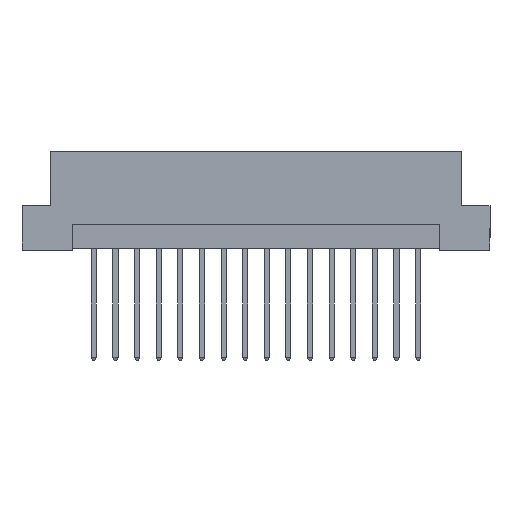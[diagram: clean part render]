
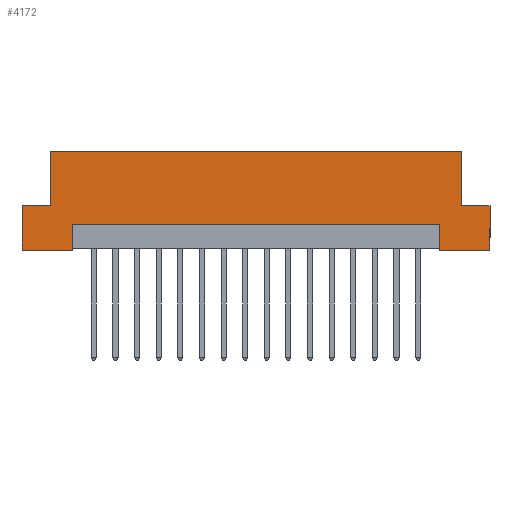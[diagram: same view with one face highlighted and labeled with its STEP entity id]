
A CAD part, front view. The second image highlights one B-rep face of the part: STEP entity #4172.
In plain terms, the highlighted planar face has unit normal (0, -1, 0).
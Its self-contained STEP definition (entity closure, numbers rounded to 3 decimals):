
#168 = CARTESIAN_POINT ( 'NONE',  ( -27.5, -4.3, 5.2 ) ) ;
#171 = VERTEX_POINT ( 'NONE', #2007 ) ;
#203 = CARTESIAN_POINT ( 'NONE',  ( 24.2, -4.3, 11.6 ) ) ;
#214 = EDGE_CURVE ( 'NONE', #5362, #229, #720, .T. ) ;
#229 = VERTEX_POINT ( 'NONE', #881 ) ;
#248 = VECTOR ( 'NONE', #6927, 1000. ) ;
#317 = CARTESIAN_POINT ( 'NONE',  ( -24.2, -4.3, 5.2 ) ) ;
#432 = EDGE_CURVE ( 'NONE', #5362, #6430, #910, .T. ) ;
#439 = ORIENTED_EDGE ( 'NONE', *, *, #6250, .T. ) ;
#578 = CARTESIAN_POINT ( 'NONE',  ( 21.6, -4.3, 0. ) ) ;
#686 = VECTOR ( 'NONE', #3645, 1000. ) ;
#720 = LINE ( 'NONE', #3054, #4377 ) ;
#773 = DIRECTION ( 'NONE',  ( 0., 0., 1. ) ) ;
#783 = LINE ( 'NONE', #5378, #5817 ) ;
#818 = PLANE ( 'NONE',  #4997 ) ;
#843 = EDGE_LOOP ( 'NONE', ( #439, #2009, #5413, #3270, #1506, #2650, #2389, #6124, #3688, #930, #3277, #5646 ) ) ;
#881 = CARTESIAN_POINT ( 'NONE',  ( 27.5, -4.3, 5.2 ) ) ;
#910 = LINE ( 'NONE', #3212, #1143 ) ;
#930 = ORIENTED_EDGE ( 'NONE', *, *, #5732, .T. ) ;
#951 = VERTEX_POINT ( 'NONE', #3939 ) ;
#1006 = CARTESIAN_POINT ( 'NONE',  ( -24.2, -4.3, 5.2 ) ) ;
#1043 = VERTEX_POINT ( 'NONE', #578 ) ;
#1130 = LINE ( 'NONE', #5734, #5064 ) ;
#1141 = LINE ( 'NONE', #3323, #6011 ) ;
#1143 = VECTOR ( 'NONE', #3805, 1000. ) ;
#1381 = VERTEX_POINT ( 'NONE', #5130 ) ;
#1394 = CARTESIAN_POINT ( 'NONE',  ( 27.5, -4.3, 0. ) ) ;
#1400 = FACE_OUTER_BOUND ( 'NONE', #843, .T. ) ;
#1461 = LINE ( 'NONE', #1394, #1472 ) ;
#1472 = VECTOR ( 'NONE', #3111, 1000. ) ;
#1506 = ORIENTED_EDGE ( 'NONE', *, *, #214, .F. ) ;
#1571 = VERTEX_POINT ( 'NONE', #1882 ) ;
#1882 = CARTESIAN_POINT ( 'NONE',  ( -24.2, -4.3, 11.6 ) ) ;
#2007 = CARTESIAN_POINT ( 'NONE',  ( -21.6, -4.3, 3. ) ) ;
#2009 = ORIENTED_EDGE ( 'NONE', *, *, #4235, .F. ) ;
#2164 = EDGE_CURVE ( 'NONE', #2628, #4800, #5532, .T. ) ;
#2256 = DIRECTION ( 'NONE',  ( 0., 0., -1. ) ) ;
#2317 = LINE ( 'NONE', #4165, #248 ) ;
#2388 = DIRECTION ( 'NONE',  ( 0., 0., -1. ) ) ;
#2389 = ORIENTED_EDGE ( 'NONE', *, *, #6824, .F. ) ;
#2508 = DIRECTION ( 'NONE',  ( 0., 0., 1. ) ) ;
#2518 = CARTESIAN_POINT ( 'NONE',  ( -21.6, -4.3, 0.2 ) ) ;
#2628 = VERTEX_POINT ( 'NONE', #168 ) ;
#2641 = LINE ( 'NONE', #2518, #4529 ) ;
#2650 = ORIENTED_EDGE ( 'NONE', *, *, #432, .T. ) ;
#2858 = EDGE_CURVE ( 'NONE', #3959, #1381, #6196, .T. ) ;
#2881 = CARTESIAN_POINT ( 'NONE',  ( 27.5, -4.3, 11.6 ) ) ;
#3054 = CARTESIAN_POINT ( 'NONE',  ( 27.5, -4.3, 5.2 ) ) ;
#3111 = DIRECTION ( 'NONE',  ( 1., 0., 0. ) ) ;
#3212 = CARTESIAN_POINT ( 'NONE',  ( 24.2, -4.3, 5.2 ) ) ;
#3270 = ORIENTED_EDGE ( 'NONE', *, *, #4976, .F. ) ;
#3272 = DIRECTION ( 'NONE',  ( 1., 0., 0. ) ) ;
#3277 = ORIENTED_EDGE ( 'NONE', *, *, #2858, .T. ) ;
#3323 = CARTESIAN_POINT ( 'NONE',  ( -27.5, -4.3, 11.6 ) ) ;
#3645 = DIRECTION ( 'NONE',  ( 1., 0., 0. ) ) ;
#3646 = EDGE_CURVE ( 'NONE', #171, #1381, #2641, .T. ) ;
#3688 = ORIENTED_EDGE ( 'NONE', *, *, #2164, .F. ) ;
#3757 = DIRECTION ( 'NONE',  ( 0., 1., 0. ) ) ;
#3801 = DIRECTION ( 'NONE',  ( 0., 0., -1. ) ) ;
#3805 = DIRECTION ( 'NONE',  ( 0., 0., 1. ) ) ;
#3939 = CARTESIAN_POINT ( 'NONE',  ( 27.5, -4.3, 0. ) ) ;
#3959 = VERTEX_POINT ( 'NONE', #7049 ) ;
#4042 = DIRECTION ( 'NONE',  ( 1., 0., 0. ) ) ;
#4060 = VERTEX_POINT ( 'NONE', #4629 ) ;
#4117 = LINE ( 'NONE', #2881, #6261 ) ;
#4165 = CARTESIAN_POINT ( 'NONE',  ( -21.6, -4.3, 3. ) ) ;
#4172 = ADVANCED_FACE ( 'NONE', ( #1400 ), #818, .F. ) ;
#4235 = EDGE_CURVE ( 'NONE', #1043, #4060, #783, .T. ) ;
#4377 = VECTOR ( 'NONE', #4668, 1000. ) ;
#4529 = VECTOR ( 'NONE', #3801, 1000. ) ;
#4629 = CARTESIAN_POINT ( 'NONE',  ( 21.6, -4.3, 3. ) ) ;
#4648 = EDGE_CURVE ( 'NONE', #4800, #1571, #5403, .T. ) ;
#4668 = DIRECTION ( 'NONE',  ( 1., 0., 0. ) ) ;
#4753 = CARTESIAN_POINT ( 'NONE',  ( 24.2, -4.3, 5.2 ) ) ;
#4800 = VERTEX_POINT ( 'NONE', #1006 ) ;
#4854 = CARTESIAN_POINT ( 'NONE',  ( 27.5, -4.3, 11.6 ) ) ;
#4976 = EDGE_CURVE ( 'NONE', #229, #951, #1130, .T. ) ;
#4997 = AXIS2_PLACEMENT_3D ( 'NONE', #4854, #3757, #6041 ) ;
#5005 = CARTESIAN_POINT ( 'NONE',  ( 27.5, -4.3, 0. ) ) ;
#5064 = VECTOR ( 'NONE', #2388, 1000. ) ;
#5130 = CARTESIAN_POINT ( 'NONE',  ( -21.6, -4.3, 0. ) ) ;
#5362 = VERTEX_POINT ( 'NONE', #4753 ) ;
#5378 = CARTESIAN_POINT ( 'NONE',  ( 21.6, -4.3, 0.2 ) ) ;
#5403 = LINE ( 'NONE', #317, #6549 ) ;
#5413 = ORIENTED_EDGE ( 'NONE', *, *, #6522, .T. ) ;
#5532 = LINE ( 'NONE', #7247, #686 ) ;
#5646 = ORIENTED_EDGE ( 'NONE', *, *, #3646, .F. ) ;
#5732 = EDGE_CURVE ( 'NONE', #2628, #3959, #1141, .T. ) ;
#5734 = CARTESIAN_POINT ( 'NONE',  ( 27.5, -4.3, 11.6 ) ) ;
#5817 = VECTOR ( 'NONE', #2508, 1000. ) ;
#6011 = VECTOR ( 'NONE', #2256, 1000. ) ;
#6041 = DIRECTION ( 'NONE',  ( -1., 0., 0. ) ) ;
#6124 = ORIENTED_EDGE ( 'NONE', *, *, #4648, .F. ) ;
#6196 = LINE ( 'NONE', #5005, #6416 ) ;
#6250 = EDGE_CURVE ( 'NONE', #171, #4060, #2317, .T. ) ;
#6261 = VECTOR ( 'NONE', #4042, 1000. ) ;
#6416 = VECTOR ( 'NONE', #3272, 1000. ) ;
#6430 = VERTEX_POINT ( 'NONE', #203 ) ;
#6522 = EDGE_CURVE ( 'NONE', #1043, #951, #1461, .T. ) ;
#6549 = VECTOR ( 'NONE', #773, 1000. ) ;
#6824 = EDGE_CURVE ( 'NONE', #1571, #6430, #4117, .T. ) ;
#6927 = DIRECTION ( 'NONE',  ( 1., 0., 0. ) ) ;
#7049 = CARTESIAN_POINT ( 'NONE',  ( -27.5, -4.3, 0. ) ) ;
#7247 = CARTESIAN_POINT ( 'NONE',  ( -27.5, -4.3, 5.2 ) ) ;
